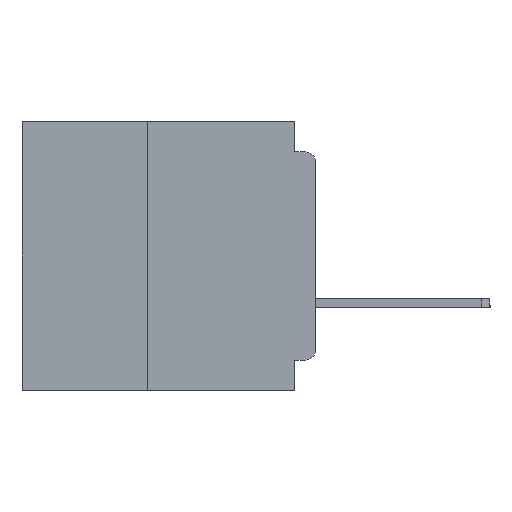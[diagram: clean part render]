
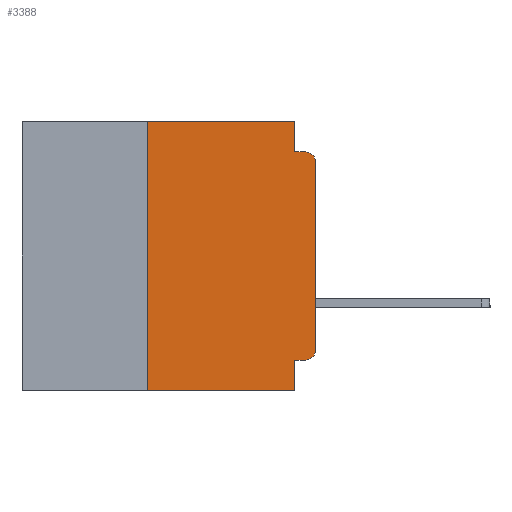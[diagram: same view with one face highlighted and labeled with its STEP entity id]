
A CAD part, left-side view. The second image highlights one B-rep face of the part: STEP entity #3388.
In plain terms, the highlighted planar face has unit normal (-1, 0, 0).
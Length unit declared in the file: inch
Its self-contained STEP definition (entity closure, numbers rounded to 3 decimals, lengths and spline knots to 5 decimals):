
#513 = CARTESIAN_POINT ( 'NONE',  ( 0., 0.031, -0.4 ) ) ;
#1453 = DIRECTION ( 'NONE',  ( 0., 0., 1. ) ) ;
#1540 = DIRECTION ( 'NONE',  ( 0., 0., -1. ) ) ;
#3388 = ADVANCED_FACE ( 'NONE', ( #14037 ), #46547, .F. ) ;
#3552 = CARTESIAN_POINT ( 'NONE',  ( 0., 0.437, -0.4 ) ) ;
#5230 = CARTESIAN_POINT ( 'NONE',  ( 0., 0., 0. ) ) ;
#5305 = DIRECTION ( 'NONE',  ( 0., -1., 0. ) ) ;
#6529 = CARTESIAN_POINT ( 'NONE',  ( 0., 0.031, -0.355 ) ) ;
#7178 = VERTEX_POINT ( 'NONE', #44629 ) ;
#7490 = EDGE_CURVE ( 'NONE', #51377, #7178, #21856, .T. ) ;
#9556 = ORIENTED_EDGE ( 'NONE', *, *, #58822, .T. ) ;
#10453 = DIRECTION ( 'NONE',  ( 0., 0., 1. ) ) ;
#13685 = CARTESIAN_POINT ( 'NONE',  ( 0., 0.015, -0.34 ) ) ;
#14037 = FACE_OUTER_BOUND ( 'NONE', #22562, .T. ) ;
#14558 = CARTESIAN_POINT ( 'NONE',  ( 0., 0.031, 0. ) ) ;
#14605 = LINE ( 'NONE', #19792, #25213 ) ;
#16907 = VERTEX_POINT ( 'NONE', #67206 ) ;
#17383 = VECTOR ( 'NONE', #10453, 39.37008 ) ;
#17390 = ORIENTED_EDGE ( 'NONE', *, *, #64395, .F. ) ;
#17447 = VERTEX_POINT ( 'NONE', #56110 ) ;
#18250 = VERTEX_POINT ( 'NONE', #66745 ) ;
#18452 = AXIS2_PLACEMENT_3D ( 'NONE', #49992, #27433, #26614 ) ;
#18571 = CARTESIAN_POINT ( 'NONE',  ( 0., 0.015, -0.045 ) ) ;
#18811 = LINE ( 'NONE', #36407, #61862 ) ;
#18894 = DIRECTION ( 'NONE',  ( 0., 0., -1. ) ) ;
#19222 = CARTESIAN_POINT ( 'NONE',  ( 0., 0., -0.355 ) ) ;
#19792 = CARTESIAN_POINT ( 'NONE',  ( 0., 0., -0.045 ) ) ;
#20010 = DIRECTION ( 'NONE',  ( 0., -1., 0. ) ) ;
#20740 = ORIENTED_EDGE ( 'NONE', *, *, #62270, .T. ) ;
#21856 = LINE ( 'NONE', #513, #61663 ) ;
#22095 = VERTEX_POINT ( 'NONE', #51801 ) ;
#22108 = EDGE_CURVE ( 'NONE', #16907, #27300, #18811, .T. ) ;
#22562 = EDGE_LOOP ( 'NONE', ( #26649, #9556, #17390, #31289, #42965, #64121, #26272, #41581, #57295, #20740 ) ) ;
#22572 = VERTEX_POINT ( 'NONE', #61086 ) ;
#24592 = LINE ( 'NONE', #63846, #64316 ) ;
#25213 = VECTOR ( 'NONE', #20010, 39.37008 ) ;
#25820 = AXIS2_PLACEMENT_3D ( 'NONE', #13685, #49981, #18894 ) ;
#26272 = ORIENTED_EDGE ( 'NONE', *, *, #51598, .T. ) ;
#26614 = DIRECTION ( 'NONE',  ( 0., 0., -1. ) ) ;
#26649 = ORIENTED_EDGE ( 'NONE', *, *, #35774, .T. ) ;
#26799 = LINE ( 'NONE', #3552, #66479 ) ;
#27300 = VERTEX_POINT ( 'NONE', #14558 ) ;
#27433 = DIRECTION ( 'NONE',  ( 1., 0., 0. ) ) ;
#27475 = CARTESIAN_POINT ( 'NONE',  ( 0., 0.031, 0. ) ) ;
#27568 = CARTESIAN_POINT ( 'NONE',  ( 0., 0.015, -0.06 ) ) ;
#31289 = ORIENTED_EDGE ( 'NONE', *, *, #48660, .F. ) ;
#32789 = DIRECTION ( 'NONE',  ( 0., 0., -1. ) ) ;
#32875 = LINE ( 'NONE', #5230, #17383 ) ;
#35774 = EDGE_CURVE ( 'NONE', #22572, #17447, #32875, .T. ) ;
#36407 = CARTESIAN_POINT ( 'NONE',  ( 0., 0.437, 0. ) ) ;
#39423 = VECTOR ( 'NONE', #1540, 39.37008 ) ;
#41581 = ORIENTED_EDGE ( 'NONE', *, *, #7490, .F. ) ;
#42082 = DIRECTION ( 'NONE',  ( 0., 0., -1. ) ) ;
#42792 = VERTEX_POINT ( 'NONE', #18571 ) ;
#42965 = ORIENTED_EDGE ( 'NONE', *, *, #22108, .F. ) ;
#44629 = CARTESIAN_POINT ( 'NONE',  ( 0., 0.031, -0.4 ) ) ;
#45077 = DIRECTION ( 'NONE',  ( 0., -1., 0. ) ) ;
#45344 = DIRECTION ( 'NONE',  ( 0., 1., 0. ) ) ;
#46284 = AXIS2_PLACEMENT_3D ( 'NONE', #27568, #63805, #32789 ) ;
#46547 = PLANE ( 'NONE',  #18452 ) ;
#48660 = EDGE_CURVE ( 'NONE', #27300, #18250, #53169, .T. ) ;
#48904 = EDGE_CURVE ( 'NONE', #22095, #51377, #64509, .T. ) ;
#49981 = DIRECTION ( 'NONE',  ( -1., 0., 0. ) ) ;
#49992 = CARTESIAN_POINT ( 'NONE',  ( 0., 0.437, 0. ) ) ;
#50149 = EDGE_CURVE ( 'NONE', #65633, #16907, #24592, .T. ) ;
#50720 = VECTOR ( 'NONE', #45344, 39.37008 ) ;
#51377 = VERTEX_POINT ( 'NONE', #6529 ) ;
#51598 = EDGE_CURVE ( 'NONE', #65633, #7178, #26799, .T. ) ;
#51801 = CARTESIAN_POINT ( 'NONE',  ( 0., 0.015, -0.355 ) ) ;
#53169 = LINE ( 'NONE', #27475, #39423 ) ;
#55899 = CIRCLE ( 'NONE', #46284, 0.015 ) ;
#56110 = CARTESIAN_POINT ( 'NONE',  ( 0., 0., -0.06 ) ) ;
#57281 = CARTESIAN_POINT ( 'NONE',  ( 0., 0.25, -0.4 ) ) ;
#57295 = ORIENTED_EDGE ( 'NONE', *, *, #48904, .F. ) ;
#57773 = CIRCLE ( 'NONE', #25820, 0.015 ) ;
#58822 = EDGE_CURVE ( 'NONE', #17447, #42792, #55899, .T. ) ;
#61086 = CARTESIAN_POINT ( 'NONE',  ( 0., 0., -0.34 ) ) ;
#61663 = VECTOR ( 'NONE', #42082, 39.37008 ) ;
#61862 = VECTOR ( 'NONE', #5305, 39.37008 ) ;
#62270 = EDGE_CURVE ( 'NONE', #22095, #22572, #57773, .T. ) ;
#63805 = DIRECTION ( 'NONE',  ( -1., 0., 0. ) ) ;
#63846 = CARTESIAN_POINT ( 'NONE',  ( 0., 0.25, -0.4 ) ) ;
#64121 = ORIENTED_EDGE ( 'NONE', *, *, #50149, .F. ) ;
#64316 = VECTOR ( 'NONE', #1453, 39.37008 ) ;
#64395 = EDGE_CURVE ( 'NONE', #18250, #42792, #14605, .T. ) ;
#64509 = LINE ( 'NONE', #19222, #50720 ) ;
#65633 = VERTEX_POINT ( 'NONE', #57281 ) ;
#66479 = VECTOR ( 'NONE', #45077, 39.37008 ) ;
#66745 = CARTESIAN_POINT ( 'NONE',  ( 0., 0.031, -0.045 ) ) ;
#67206 = CARTESIAN_POINT ( 'NONE',  ( 0., 0.25, 0. ) ) ;
